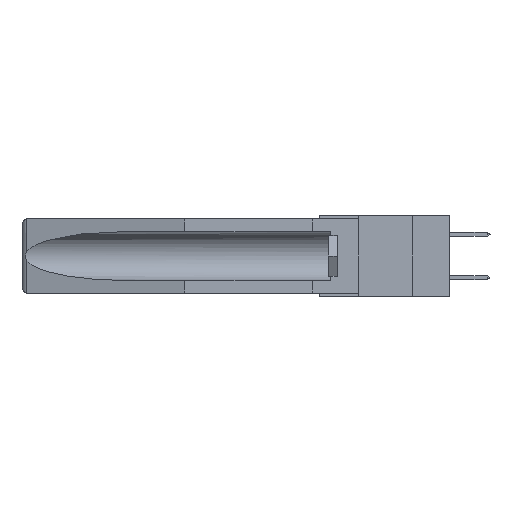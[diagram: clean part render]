
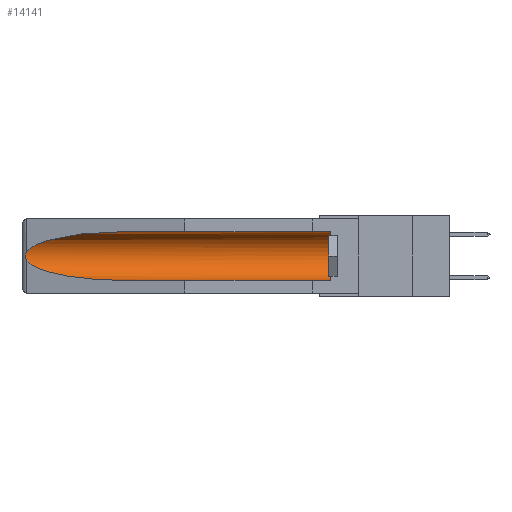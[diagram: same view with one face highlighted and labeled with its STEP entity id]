
A CAD part, left-side view. The second image highlights one B-rep face of the part: STEP entity #14141.
In plain terms, the highlighted cylindrical face has radius 2.857 mm (diameter 5.715 mm), a partial arc.
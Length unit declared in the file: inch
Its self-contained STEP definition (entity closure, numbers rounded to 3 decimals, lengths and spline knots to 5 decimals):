
#171 = DIRECTION ( 'NONE',  ( 0., 1., 0. ) ) ;
#707 = CARTESIAN_POINT ( 'NONE',  ( 0.25451, 1.48313, -0.09465 ) ) ;
#1165 = AXIS2_PLACEMENT_3D ( 'NONE', #17781, #171, #5480 ) ;
#1428 = CARTESIAN_POINT ( 'NONE',  ( 0.26537, 1.52718, -0.14972 ) ) ;
#1453 = CARTESIAN_POINT ( 'NONE',  ( 0.155, 0.126, -0.059 ) ) ;
#1586 = VERTEX_POINT ( 'NONE', #9129 ) ;
#2429 = ORIENTED_EDGE ( 'NONE', *, *, #16249, .T. ) ;
#2515 = CARTESIAN_POINT ( 'NONE',  ( 0.155, 1.07973, -0.284 ) ) ;
#2622 = VERTEX_POINT ( 'NONE', #1453 ) ;
#3244 = ORIENTED_EDGE ( 'NONE', *, *, #8713, .T. ) ;
#3727 = VERTEX_POINT ( 'NONE', #10120 ) ;
#4948 = CARTESIAN_POINT ( 'NONE',  ( 0.26537, 1.52718, -0.19328 ) ) ;
#4992 = ORIENTED_EDGE ( 'NONE', *, *, #17880, .F. ) ;
#5480 = DIRECTION ( 'NONE',  ( 0., 0., 1. ) ) ;
#5950 = EDGE_CURVE ( 'NONE', #1586, #18983, #11230, .T. ) ;
#6129 = CARTESIAN_POINT ( 'NONE',  ( 0.26537, 1.52718, -0.14972 ) ) ;
#6622 = CARTESIAN_POINT ( 'NONE',  ( 0.26655, 1.53094, -0.18657 ) ) ;
#6697 = CARTESIAN_POINT ( 'NONE',  ( 0.26597, 1.52961, -0.15275 ) ) ;
#6971 = ORIENTED_EDGE ( 'NONE', *, *, #17123, .T. ) ;
#7107 =( BOUNDED_CURVE ( )  B_SPLINE_CURVE ( 3, ( #16721, #20202, #18189, #2515 ),
 .UNSPECIFIED., .F., .F. ) 
 B_SPLINE_CURVE_WITH_KNOTS ( ( 4, 4 ),
 ( 0.1948, 1.5708 ),
 .UNSPECIFIED. ) 
 CURVE ( )  GEOMETRIC_REPRESENTATION_ITEM ( )  RATIONAL_B_SPLINE_CURVE ( ( 1., 0.848, 0.848, 1. ) ) 
 REPRESENTATION_ITEM ( '' )  );
#8006 = LINE ( 'NONE', #8495, #12174 ) ;
#8148 = CYLINDRICAL_SURFACE ( 'NONE', #1165, 0.1125 ) ;
#8331 = CARTESIAN_POINT ( 'NONE',  ( 0.26597, 1.5296, -0.19026 ) ) ;
#8495 = CARTESIAN_POINT ( 'NONE',  ( 0.155, -0.30754, -0.059 ) ) ;
#8713 = EDGE_CURVE ( 'NONE', #3727, #2622, #11557, .T. ) ;
#9129 = CARTESIAN_POINT ( 'NONE',  ( 0.26537, 1.52718, -0.14972 ) ) ;
#9691 = DIRECTION ( 'NONE',  ( 0., 0., 1. ) ) ;
#9767 = CARTESIAN_POINT ( 'NONE',  ( 0.155, 0.126, -0.1715 ) ) ;
#10067 = ORIENTED_EDGE ( 'NONE', *, *, #5950, .T. ) ;
#10120 = CARTESIAN_POINT ( 'NONE',  ( 0.155, 0.126, -0.284 ) ) ;
#10598 = CARTESIAN_POINT ( 'NONE',  ( 0.155, 1.07973, -0.284 ) ) ;
#10905 = FACE_OUTER_BOUND ( 'NONE', #17181, .T. ) ;
#11079 = CARTESIAN_POINT ( 'NONE',  ( 0.155, -0.30754, -0.284 ) ) ;
#11135 = ORIENTED_EDGE ( 'NONE', *, *, #19209, .T. ) ;
#11230 = B_SPLINE_CURVE_WITH_KNOTS ( 'NONE', 3,
 ( #1428, #6697, #15485, #17255, #22774, #15559, #17551, #6622, #8331, #4948 ),
 .UNSPECIFIED., .F., .F.,
 ( 4, 2, 2, 2, 4 ),
 ( 0., 0.00029, 0.00058, 0.00087, 0.00117 ),
 .UNSPECIFIED. ) ;
#11385 = VERTEX_POINT ( 'NONE', #10598 ) ;
#11523 = LINE ( 'NONE', #11079, #20961 ) ;
#11557 = CIRCLE ( 'NONE', #19366, 0.1125 ) ;
#11640 = CARTESIAN_POINT ( 'NONE',  ( 0.21114, 1.30732, -0.059 ) ) ;
#12174 = VECTOR ( 'NONE', #22640, 39.37008 ) ;
#14141 = ADVANCED_FACE ( 'NONE', ( #10905 ), #8148, .F. ) ;
#14635 = CARTESIAN_POINT ( 'NONE',  ( 0.155, 1.07973, -0.059 ) ) ;
#15107 =( BOUNDED_CURVE ( )  B_SPLINE_CURVE ( 3, ( #20245, #11640, #707, #6129 ),
 .UNSPECIFIED., .F., .F. ) 
 B_SPLINE_CURVE_WITH_KNOTS ( ( 4, 4 ),
 ( 4.71239, 6.08839 ),
 .UNSPECIFIED. ) 
 CURVE ( )  GEOMETRIC_REPRESENTATION_ITEM ( )  RATIONAL_B_SPLINE_CURVE ( ( 1., 0.848, 0.848, 1. ) ) 
 REPRESENTATION_ITEM ( '' )  );
#15379 = CARTESIAN_POINT ( 'NONE',  ( 0.26537, 1.52718, -0.19328 ) ) ;
#15485 = CARTESIAN_POINT ( 'NONE',  ( 0.26654, 1.53092, -0.15636 ) ) ;
#15559 = CARTESIAN_POINT ( 'NONE',  ( 0.2675, 1.53308, -0.17534 ) ) ;
#16249 = EDGE_CURVE ( 'NONE', #17466, #1586, #15107, .T. ) ;
#16721 = CARTESIAN_POINT ( 'NONE',  ( 0.26537, 1.52718, -0.19328 ) ) ;
#17123 = EDGE_CURVE ( 'NONE', #2622, #17466, #8006, .T. ) ;
#17181 = EDGE_LOOP ( 'NONE', ( #2429, #10067, #11135, #4992, #3244, #6971 ) ) ;
#17255 = CARTESIAN_POINT ( 'NONE',  ( 0.2673, 1.5327, -0.16383 ) ) ;
#17466 = VERTEX_POINT ( 'NONE', #14635 ) ;
#17551 = CARTESIAN_POINT ( 'NONE',  ( 0.2673, 1.53269, -0.17917 ) ) ;
#17781 = CARTESIAN_POINT ( 'NONE',  ( 0.155, -0.30754, -0.1715 ) ) ;
#17880 = EDGE_CURVE ( 'NONE', #3727, #11385, #11523, .T. ) ;
#18189 = CARTESIAN_POINT ( 'NONE',  ( 0.21114, 1.30732, -0.284 ) ) ;
#18983 = VERTEX_POINT ( 'NONE', #15379 ) ;
#19209 = EDGE_CURVE ( 'NONE', #18983, #11385, #7107, .T. ) ;
#19366 = AXIS2_PLACEMENT_3D ( 'NONE', #9767, #22212, #9691 ) ;
#19929 = DIRECTION ( 'NONE',  ( 0., 1., 0. ) ) ;
#20202 = CARTESIAN_POINT ( 'NONE',  ( 0.25451, 1.48313, -0.24835 ) ) ;
#20245 = CARTESIAN_POINT ( 'NONE',  ( 0.155, 1.07973, -0.059 ) ) ;
#20961 = VECTOR ( 'NONE', #19929, 39.37008 ) ;
#22212 = DIRECTION ( 'NONE',  ( 0., -1., 0. ) ) ;
#22640 = DIRECTION ( 'NONE',  ( 0., 1., 0. ) ) ;
#22774 = CARTESIAN_POINT ( 'NONE',  ( 0.2675, 1.53308, -0.16763 ) ) ;
